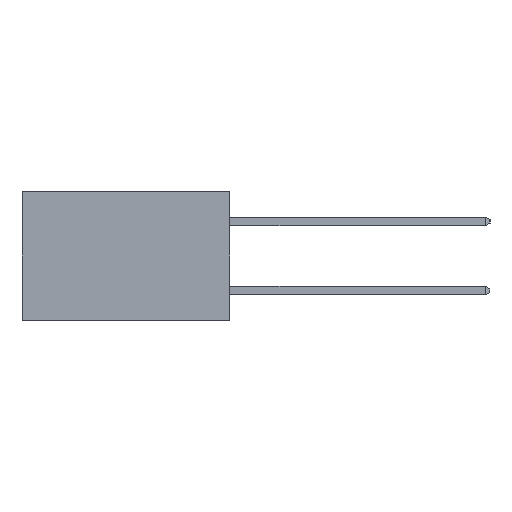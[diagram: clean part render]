
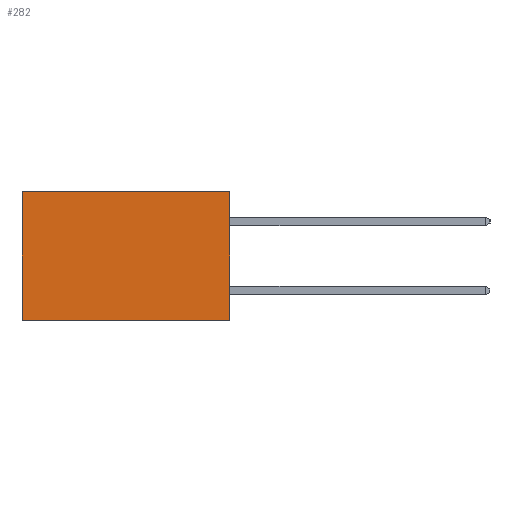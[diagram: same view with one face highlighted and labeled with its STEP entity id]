
A CAD part, left-side view. The second image highlights one B-rep face of the part: STEP entity #282.
In plain terms, the highlighted planar face has unit normal (-1, 0, 0).
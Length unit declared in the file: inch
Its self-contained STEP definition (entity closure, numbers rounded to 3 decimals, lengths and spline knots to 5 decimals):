
#282 = ADVANCED_FACE ( 'NONE', ( #13100 ), #5740, .F. ) ;
#357 = AXIS2_PLACEMENT_3D ( 'NONE', #1343, #10776, #3123 ) ;
#1343 = CARTESIAN_POINT ( 'NONE',  ( 0.298, 0., 0. ) ) ;
#2590 = LINE ( 'NONE', #15338, #11870 ) ;
#3002 = LINE ( 'NONE', #15519, #14978 ) ;
#3123 = DIRECTION ( 'NONE',  ( 0., 0., -1. ) ) ;
#4363 = DIRECTION ( 'NONE',  ( 0., 1., 0. ) ) ;
#4791 = VECTOR ( 'NONE', #6609, 39.37008 ) ;
#4882 = CARTESIAN_POINT ( 'NONE',  ( 0.298, 0.6, 0. ) ) ;
#5597 = VECTOR ( 'NONE', #4363, 39.37008 ) ;
#5740 = PLANE ( 'NONE',  #357 ) ;
#6221 = EDGE_CURVE ( 'NONE', #13985, #12997, #3002, .T. ) ;
#6609 = DIRECTION ( 'NONE',  ( 0., 0., -1. ) ) ;
#7098 = ORIENTED_EDGE ( 'NONE', *, *, #6221, .T. ) ;
#7378 = EDGE_LOOP ( 'NONE', ( #11473, #7748, #8995, #7098 ) ) ;
#7748 = ORIENTED_EDGE ( 'NONE', *, *, #11420, .F. ) ;
#7769 = VERTEX_POINT ( 'NONE', #15616 ) ;
#8214 = LINE ( 'NONE', #10390, #4791 ) ;
#8995 = ORIENTED_EDGE ( 'NONE', *, *, #11440, .F. ) ;
#9458 = CARTESIAN_POINT ( 'NONE',  ( 0.298, 0., -0.37 ) ) ;
#10221 = LINE ( 'NONE', #9458, #5597 ) ;
#10390 = CARTESIAN_POINT ( 'NONE',  ( 0.298, 0.6, 0. ) ) ;
#10776 = DIRECTION ( 'NONE',  ( 1., 0., 0. ) ) ;
#11420 = EDGE_CURVE ( 'NONE', #13597, #7769, #10221, .T. ) ;
#11440 = EDGE_CURVE ( 'NONE', #13985, #13597, #2590, .T. ) ;
#11473 = ORIENTED_EDGE ( 'NONE', *, *, #14194, .T. ) ;
#11780 = CARTESIAN_POINT ( 'NONE',  ( 0.298, 0., -0.37 ) ) ;
#11870 = VECTOR ( 'NONE', #14229, 39.37008 ) ;
#12997 = VERTEX_POINT ( 'NONE', #4882 ) ;
#13100 = FACE_OUTER_BOUND ( 'NONE', #7378, .T. ) ;
#13509 = CARTESIAN_POINT ( 'NONE',  ( 0.298, 0., 0. ) ) ;
#13597 = VERTEX_POINT ( 'NONE', #11780 ) ;
#13985 = VERTEX_POINT ( 'NONE', #13509 ) ;
#14194 = EDGE_CURVE ( 'NONE', #12997, #7769, #8214, .T. ) ;
#14229 = DIRECTION ( 'NONE',  ( 0., 0., -1. ) ) ;
#14978 = VECTOR ( 'NONE', #15103, 39.37008 ) ;
#15103 = DIRECTION ( 'NONE',  ( 0., 1., 0. ) ) ;
#15338 = CARTESIAN_POINT ( 'NONE',  ( 0.298, 0., 0. ) ) ;
#15519 = CARTESIAN_POINT ( 'NONE',  ( 0.298, 0., 0. ) ) ;
#15616 = CARTESIAN_POINT ( 'NONE',  ( 0.298, 0.6, -0.37 ) ) ;
